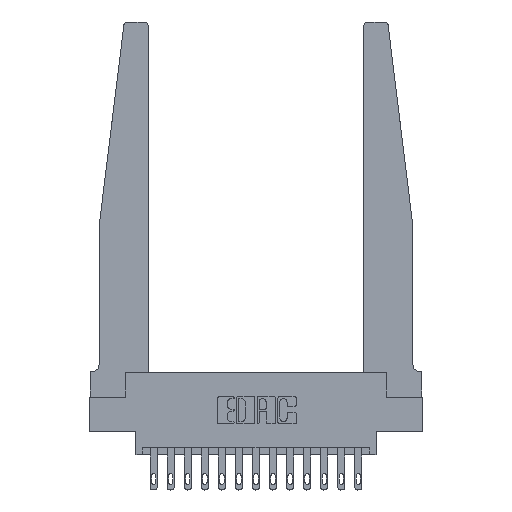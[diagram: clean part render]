
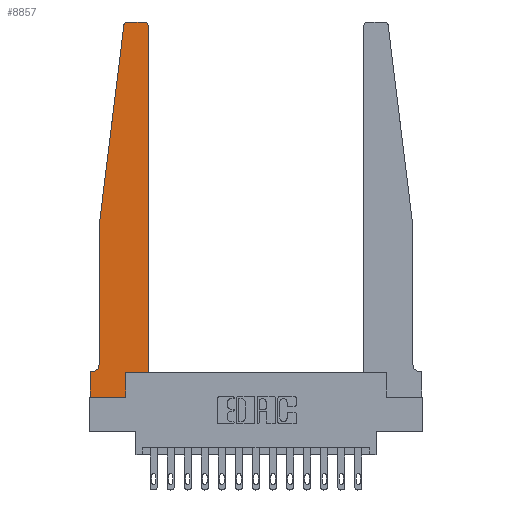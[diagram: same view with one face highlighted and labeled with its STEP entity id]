
A CAD part, top view. The second image highlights one B-rep face of the part: STEP entity #8857.
In plain terms, the highlighted planar face has unit normal (0, 0, 1).
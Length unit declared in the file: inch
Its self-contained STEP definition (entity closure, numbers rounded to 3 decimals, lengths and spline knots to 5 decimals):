
#175 = EDGE_CURVE ( 'NONE', #2076, #4276, #11654, .T. ) ;
#427 = EDGE_CURVE ( 'NONE', #9308, #9412, #9721, .T. ) ;
#926 = EDGE_CURVE ( 'NONE', #2545, #9308, #9916, .T. ) ;
#1097 = VERTEX_POINT ( 'NONE', #16998 ) ;
#1182 = ORIENTED_EDGE ( 'NONE', *, *, #10660, .T. ) ;
#1723 = DIRECTION ( 'NONE',  ( 0., 0., 1. ) ) ;
#1738 = VERTEX_POINT ( 'NONE', #2804 ) ;
#1743 = DIRECTION ( 'NONE',  ( 0., 1., 0. ) ) ;
#1984 = AXIS2_PLACEMENT_3D ( 'NONE', #4045, #3689, #7735 ) ;
#2076 = VERTEX_POINT ( 'NONE', #2596 ) ;
#2156 = DIRECTION ( 'NONE',  ( 1., 0., 0. ) ) ;
#2336 = ORIENTED_EDGE ( 'NONE', *, *, #4660, .T. ) ;
#2545 = VERTEX_POINT ( 'NONE', #3553 ) ;
#2596 = CARTESIAN_POINT ( 'NONE',  ( 0.27653, 2.75, 0.37 ) ) ;
#2608 = VERTEX_POINT ( 'NONE', #6701 ) ;
#2804 = CARTESIAN_POINT ( 'NONE',  ( 0.2605, 0., 0.37 ) ) ;
#3229 = LINE ( 'NONE', #10313, #4043 ) ;
#3361 = EDGE_CURVE ( 'NONE', #2608, #1738, #3229, .T. ) ;
#3389 = PLANE ( 'NONE',  #4714 ) ;
#3391 = VERTEX_POINT ( 'NONE', #7636 ) ;
#3424 = ORIENTED_EDGE ( 'NONE', *, *, #7313, .T. ) ;
#3553 = CARTESIAN_POINT ( 'NONE',  ( 0.425, 0.18, 0.37 ) ) ;
#3689 = DIRECTION ( 'NONE',  ( 0., 0., 1. ) ) ;
#3691 = AXIS2_PLACEMENT_3D ( 'NONE', #8455, #1723, #7018 ) ;
#3786 = DIRECTION ( 'NONE',  ( -1., 0., 0. ) ) ;
#4013 = VECTOR ( 'NONE', #1743, 39.37008 ) ;
#4043 = VECTOR ( 'NONE', #2156, 39.37008 ) ;
#4045 = CARTESIAN_POINT ( 'NONE',  ( 0.395, 2.72, 0.37 ) ) ;
#4091 = CARTESIAN_POINT ( 'NONE',  ( 0.2605, 0.18, 0.37 ) ) ;
#4276 = VERTEX_POINT ( 'NONE', #7646 ) ;
#4551 = ORIENTED_EDGE ( 'NONE', *, *, #427, .T. ) ;
#4660 = EDGE_CURVE ( 'NONE', #16301, #1097, #8116, .T. ) ;
#4714 = AXIS2_PLACEMENT_3D ( 'NONE', #15715, #14541, #17217 ) ;
#4806 = CARTESIAN_POINT ( 'NONE',  ( 0.425, 2.72, 0.37 ) ) ;
#5119 = CARTESIAN_POINT ( 'NONE',  ( 0.25, 2.75, 0.37 ) ) ;
#5178 = CARTESIAN_POINT ( 'NONE',  ( 0.065, 0.1875, 0.37 ) ) ;
#5396 = ORIENTED_EDGE ( 'NONE', *, *, #14355, .T. ) ;
#6357 = DIRECTION ( 'NONE',  ( -1., 0., 0. ) ) ;
#6474 = VECTOR ( 'NONE', #9315, 39.37008 ) ;
#6533 = ORIENTED_EDGE ( 'NONE', *, *, #10707, .T. ) ;
#6701 = CARTESIAN_POINT ( 'NONE',  ( 0., 0., 0.37 ) ) ;
#7018 = DIRECTION ( 'NONE',  ( 1., 0., 0. ) ) ;
#7313 = EDGE_CURVE ( 'NONE', #1097, #16256, #13297, .T. ) ;
#7343 = ORIENTED_EDGE ( 'NONE', *, *, #17463, .T. ) ;
#7636 = CARTESIAN_POINT ( 'NONE',  ( 0.2605, 0.18, 0.37 ) ) ;
#7646 = CARTESIAN_POINT ( 'NONE',  ( 0.24675, 2.72367, 0.37 ) ) ;
#7735 = DIRECTION ( 'NONE',  ( 1., 0., 0. ) ) ;
#7782 = LINE ( 'NONE', #10375, #8538 ) ;
#7958 = ORIENTED_EDGE ( 'NONE', *, *, #175, .T. ) ;
#7968 = LINE ( 'NONE', #4091, #6474 ) ;
#8080 = EDGE_CURVE ( 'NONE', #4276, #14239, #13066, .T. ) ;
#8116 = CIRCLE ( 'NONE', #17171, 0.05 ) ;
#8269 = ORIENTED_EDGE ( 'NONE', *, *, #3361, .T. ) ;
#8321 = LINE ( 'NONE', #14871, #17266 ) ;
#8393 = CARTESIAN_POINT ( 'NONE',  ( 0.065, 0.2375, 0.37 ) ) ;
#8455 = CARTESIAN_POINT ( 'NONE',  ( 0.27653, 2.72, 0.37 ) ) ;
#8538 = VECTOR ( 'NONE', #15800, 39.37008 ) ;
#8857 = ADVANCED_FACE ( 'NONE', ( #12760 ), #3389, .T. ) ;
#8924 = DIRECTION ( 'NONE',  ( -0.122, -0.992, 0. ) ) ;
#9308 = VERTEX_POINT ( 'NONE', #4806 ) ;
#9315 = DIRECTION ( 'NONE',  ( 0., 1., 0. ) ) ;
#9412 = VERTEX_POINT ( 'NONE', #9488 ) ;
#9488 = CARTESIAN_POINT ( 'NONE',  ( 0.395, 2.75, 0.37 ) ) ;
#9494 = DIRECTION ( 'NONE',  ( 0., -1., 0. ) ) ;
#9721 = CIRCLE ( 'NONE', #1984, 0.03 ) ;
#9916 = LINE ( 'NONE', #15135, #4013 ) ;
#10313 = CARTESIAN_POINT ( 'NONE',  ( 0., 0., 0.37 ) ) ;
#10348 = ORIENTED_EDGE ( 'NONE', *, *, #16480, .T. ) ;
#10375 = CARTESIAN_POINT ( 'NONE',  ( 0., 0., 0.37 ) ) ;
#10424 = CARTESIAN_POINT ( 'NONE',  ( 0.065, 1.25, 0.37 ) ) ;
#10626 = LINE ( 'NONE', #11940, #16426 ) ;
#10648 = DIRECTION ( 'NONE',  ( -1., 0., 0. ) ) ;
#10660 = EDGE_CURVE ( 'NONE', #1738, #3391, #7968, .T. ) ;
#10707 = EDGE_CURVE ( 'NONE', #3391, #2545, #10626, .T. ) ;
#10732 = EDGE_LOOP ( 'NONE', ( #10348, #7958, #12401, #7343, #2336, #3424, #5396, #8269, #1182, #6533, #15830, #4551 ) ) ;
#10801 = CARTESIAN_POINT ( 'NONE',  ( 0., 0.1875, 0.37 ) ) ;
#11654 = CIRCLE ( 'NONE', #3691, 0.03 ) ;
#11940 = CARTESIAN_POINT ( 'NONE',  ( 0.425, 0.18, 0.37 ) ) ;
#12401 = ORIENTED_EDGE ( 'NONE', *, *, #8080, .T. ) ;
#12760 = FACE_OUTER_BOUND ( 'NONE', #10732, .T. ) ;
#13066 = LINE ( 'NONE', #10424, #15824 ) ;
#13297 = LINE ( 'NONE', #5178, #14637 ) ;
#14239 = VERTEX_POINT ( 'NONE', #15168 ) ;
#14355 = EDGE_CURVE ( 'NONE', #16256, #2608, #7782, .T. ) ;
#14541 = DIRECTION ( 'NONE',  ( 0., 0., 1. ) ) ;
#14637 = VECTOR ( 'NONE', #10648, 39.37008 ) ;
#14871 = CARTESIAN_POINT ( 'NONE',  ( 0.065, 1.25, 0.37 ) ) ;
#15135 = CARTESIAN_POINT ( 'NONE',  ( 0.425, 0.18, 0.37 ) ) ;
#15168 = CARTESIAN_POINT ( 'NONE',  ( 0.065, 1.25, 0.37 ) ) ;
#15536 = DIRECTION ( 'NONE',  ( 0., 0., -1. ) ) ;
#15715 = CARTESIAN_POINT ( 'NONE',  ( 0., 0.1875, 0.37 ) ) ;
#15800 = DIRECTION ( 'NONE',  ( 0., -1., 0. ) ) ;
#15824 = VECTOR ( 'NONE', #8924, 39.37008 ) ;
#15826 = VECTOR ( 'NONE', #3786, 39.37008 ) ;
#15830 = ORIENTED_EDGE ( 'NONE', *, *, #926, .T. ) ;
#15894 = CARTESIAN_POINT ( 'NONE',  ( 0.015, 0.2375, 0.37 ) ) ;
#16256 = VERTEX_POINT ( 'NONE', #10801 ) ;
#16301 = VERTEX_POINT ( 'NONE', #8393 ) ;
#16426 = VECTOR ( 'NONE', #17387, 39.37008 ) ;
#16480 = EDGE_CURVE ( 'NONE', #9412, #2076, #16891, .T. ) ;
#16891 = LINE ( 'NONE', #5119, #15826 ) ;
#16998 = CARTESIAN_POINT ( 'NONE',  ( 0.015, 0.1875, 0.37 ) ) ;
#17171 = AXIS2_PLACEMENT_3D ( 'NONE', #15894, #15536, #6357 ) ;
#17217 = DIRECTION ( 'NONE',  ( 1., 0., 0. ) ) ;
#17266 = VECTOR ( 'NONE', #9494, 39.37008 ) ;
#17387 = DIRECTION ( 'NONE',  ( 1., 0., 0. ) ) ;
#17463 = EDGE_CURVE ( 'NONE', #14239, #16301, #8321, .T. ) ;
